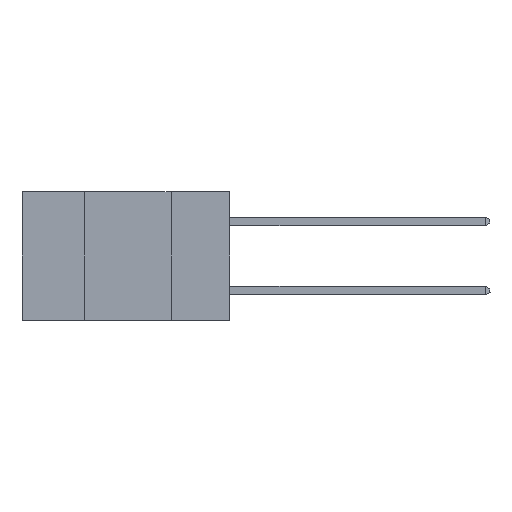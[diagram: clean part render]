
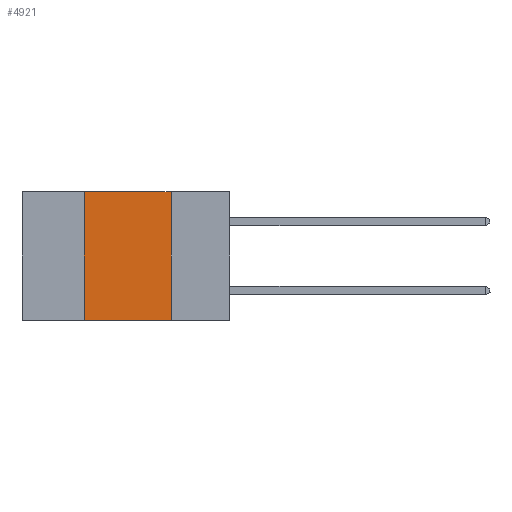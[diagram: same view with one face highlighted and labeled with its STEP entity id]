
A CAD part, left-side view. The second image highlights one B-rep face of the part: STEP entity #4921.
In plain terms, the highlighted planar face has unit normal (-1, 0, 0).
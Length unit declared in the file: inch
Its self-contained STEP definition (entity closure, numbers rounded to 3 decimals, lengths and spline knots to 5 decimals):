
#29 = LINE ( 'NONE', #18298, #16828 ) ;
#273 = DIRECTION ( 'NONE',  ( 0., -1., 0. ) ) ;
#496 = AXIS2_PLACEMENT_3D ( 'NONE', #7269, #14230, #10006 ) ;
#602 = LINE ( 'NONE', #12745, #8344 ) ;
#829 = CARTESIAN_POINT ( 'NONE',  ( 0., 0.17, 0. ) ) ;
#1004 = LINE ( 'NONE', #7111, #14286 ) ;
#1804 = VECTOR ( 'NONE', #7314, 39.37008 ) ;
#2342 = ORIENTED_EDGE ( 'NONE', *, *, #15422, .F. ) ;
#2725 = CARTESIAN_POINT ( 'NONE',  ( 0., 0.42, -0.37 ) ) ;
#3279 = EDGE_LOOP ( 'NONE', ( #2342, #11020, #12633, #17233 ) ) ;
#4921 = ADVANCED_FACE ( 'NONE', ( #5068 ), #5968, .F. ) ;
#5068 = FACE_OUTER_BOUND ( 'NONE', #3279, .T. ) ;
#5968 = PLANE ( 'NONE',  #496 ) ;
#6076 = EDGE_CURVE ( 'NONE', #18125, #17310, #602, .T. ) ;
#6373 = VERTEX_POINT ( 'NONE', #8400 ) ;
#7111 = CARTESIAN_POINT ( 'NONE',  ( 0., 0.6, 0. ) ) ;
#7269 = CARTESIAN_POINT ( 'NONE',  ( 0., 0.6, 0. ) ) ;
#7289 = VERTEX_POINT ( 'NONE', #829 ) ;
#7314 = DIRECTION ( 'NONE',  ( 0., 0., 1. ) ) ;
#8261 = CARTESIAN_POINT ( 'NONE',  ( 0., 0.17, -0.37 ) ) ;
#8344 = VECTOR ( 'NONE', #18227, 39.37008 ) ;
#8400 = CARTESIAN_POINT ( 'NONE',  ( 0., 0.42, 0. ) ) ;
#9882 = DIRECTION ( 'NONE',  ( 0., 0., -1. ) ) ;
#10006 = DIRECTION ( 'NONE',  ( 0., 0., -1. ) ) ;
#11020 = ORIENTED_EDGE ( 'NONE', *, *, #12802, .F. ) ;
#12633 = ORIENTED_EDGE ( 'NONE', *, *, #17842, .F. ) ;
#12658 = LINE ( 'NONE', #14388, #1804 ) ;
#12745 = CARTESIAN_POINT ( 'NONE',  ( 0., 0.6, -0.37 ) ) ;
#12802 = EDGE_CURVE ( 'NONE', #6373, #7289, #1004, .T. ) ;
#14230 = DIRECTION ( 'NONE',  ( 1., 0., 0. ) ) ;
#14286 = VECTOR ( 'NONE', #273, 39.37008 ) ;
#14388 = CARTESIAN_POINT ( 'NONE',  ( 0., 0.42, 0. ) ) ;
#15422 = EDGE_CURVE ( 'NONE', #7289, #17310, #29, .T. ) ;
#16828 = VECTOR ( 'NONE', #9882, 39.37008 ) ;
#17233 = ORIENTED_EDGE ( 'NONE', *, *, #6076, .T. ) ;
#17310 = VERTEX_POINT ( 'NONE', #8261 ) ;
#17842 = EDGE_CURVE ( 'NONE', #18125, #6373, #12658, .T. ) ;
#18125 = VERTEX_POINT ( 'NONE', #2725 ) ;
#18227 = DIRECTION ( 'NONE',  ( 0., -1., 0. ) ) ;
#18298 = CARTESIAN_POINT ( 'NONE',  ( 0., 0.17, 0. ) ) ;
